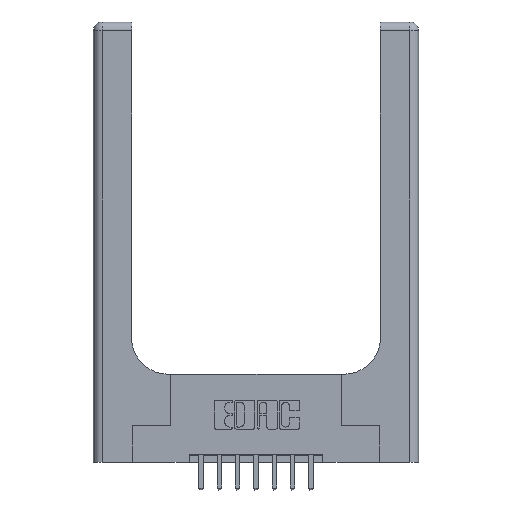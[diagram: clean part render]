
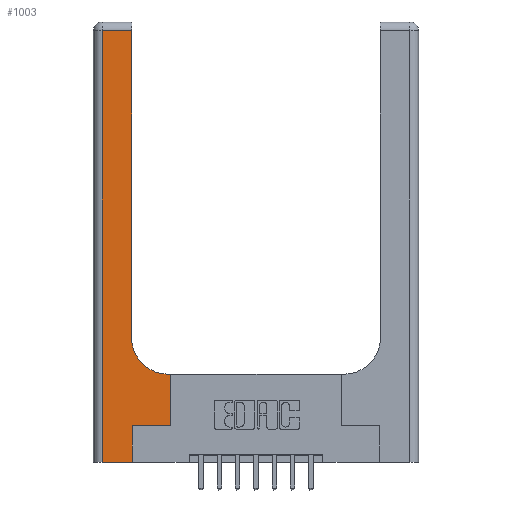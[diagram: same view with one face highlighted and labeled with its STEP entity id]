
A CAD part, top view. The second image highlights one B-rep face of the part: STEP entity #1003.
In plain terms, the highlighted planar face has unit normal (0, 0, 1).
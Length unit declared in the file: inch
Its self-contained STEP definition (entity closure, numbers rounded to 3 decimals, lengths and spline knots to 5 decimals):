
#156 = CARTESIAN_POINT ( 'NONE',  ( 0.51, 0.85, 0.37 ) ) ;
#157 = LINE ( 'NONE', #9259, #11962 ) ;
#174 = VECTOR ( 'NONE', #3947, 39.37008 ) ;
#185 = DIRECTION ( 'NONE',  ( 0., 1., 0. ) ) ;
#489 = VERTEX_POINT ( 'NONE', #7079 ) ;
#1003 = ADVANCED_FACE ( 'NONE', ( #2369 ), #7775, .F. ) ;
#1210 = CARTESIAN_POINT ( 'NONE',  ( 0.265, 0.25, 0.37 ) ) ;
#1618 = LINE ( 'NONE', #1210, #6389 ) ;
#1628 = EDGE_CURVE ( 'NONE', #11171, #5845, #3055, .T. ) ;
#1662 = VERTEX_POINT ( 'NONE', #12021 ) ;
#1709 = DIRECTION ( 'NONE',  ( 0., -1., 0. ) ) ;
#1974 = DIRECTION ( 'NONE',  ( 1., 0., 0. ) ) ;
#2057 = CARTESIAN_POINT ( 'NONE',  ( 0.51, 0.6, 0.37 ) ) ;
#2179 = VECTOR ( 'NONE', #1974, 39.37008 ) ;
#2369 = FACE_OUTER_BOUND ( 'NONE', #11499, .T. ) ;
#2443 = DIRECTION ( 'NONE',  ( 1., 0., 0. ) ) ;
#2657 = LINE ( 'NONE', #5059, #6920 ) ;
#2875 = LINE ( 'NONE', #8528, #2179 ) ;
#2930 = LINE ( 'NONE', #10883, #8245 ) ;
#3055 = LINE ( 'NONE', #8002, #6440 ) ;
#3266 = VERTEX_POINT ( 'NONE', #8598 ) ;
#3276 = CARTESIAN_POINT ( 'NONE',  ( 0., 3., 0.37 ) ) ;
#3330 = ORIENTED_EDGE ( 'NONE', *, *, #7799, .T. ) ;
#3516 = EDGE_CURVE ( 'NONE', #12905, #3266, #2657, .T. ) ;
#3571 = ORIENTED_EDGE ( 'NONE', *, *, #1628, .T. ) ;
#3836 = ORIENTED_EDGE ( 'NONE', *, *, #6866, .T. ) ;
#3947 = DIRECTION ( 'NONE',  ( -1., 0., 0. ) ) ;
#4151 = CARTESIAN_POINT ( 'NONE',  ( 0., 2.94, 0.37 ) ) ;
#4368 = DIRECTION ( 'NONE',  ( 0., 1., 0. ) ) ;
#4957 = LINE ( 'NONE', #4151, #174 ) ;
#5059 = CARTESIAN_POINT ( 'NONE',  ( 0.06, 3., 0.37 ) ) ;
#5617 = VERTEX_POINT ( 'NONE', #11482 ) ;
#5618 = DIRECTION ( 'NONE',  ( 1., 0., 0. ) ) ;
#5726 = VERTEX_POINT ( 'NONE', #13419 ) ;
#5845 = VERTEX_POINT ( 'NONE', #13540 ) ;
#6379 = EDGE_CURVE ( 'NONE', #3266, #5617, #2875, .T. ) ;
#6389 = VECTOR ( 'NONE', #5618, 39.37008 ) ;
#6440 = VECTOR ( 'NONE', #185, 39.37008 ) ;
#6866 = EDGE_CURVE ( 'NONE', #489, #9296, #9216, .T. ) ;
#6920 = VECTOR ( 'NONE', #1709, 39.37008 ) ;
#7079 = CARTESIAN_POINT ( 'NONE',  ( 0.528, 0.6, 0.37 ) ) ;
#7583 = EDGE_CURVE ( 'NONE', #5726, #1662, #1618, .T. ) ;
#7775 = PLANE ( 'NONE',  #13805 ) ;
#7799 = EDGE_CURVE ( 'NONE', #5845, #12905, #4957, .T. ) ;
#7831 = VECTOR ( 'NONE', #9234, 39.37008 ) ;
#8002 = CARTESIAN_POINT ( 'NONE',  ( 0.26, 3., 0.37 ) ) ;
#8194 = EDGE_CURVE ( 'NONE', #5617, #5726, #157, .T. ) ;
#8245 = VECTOR ( 'NONE', #4368, 39.37008 ) ;
#8502 = CARTESIAN_POINT ( 'NONE',  ( 0.26, 0.85, 0.37 ) ) ;
#8528 = CARTESIAN_POINT ( 'NONE',  ( 0., 0., 0.37 ) ) ;
#8598 = CARTESIAN_POINT ( 'NONE',  ( 0.06, 0., 0.37 ) ) ;
#9134 = CIRCLE ( 'NONE', #13673, 0.25 ) ;
#9216 = LINE ( 'NONE', #11328, #7831 ) ;
#9234 = DIRECTION ( 'NONE',  ( -1., 0., 0. ) ) ;
#9259 = CARTESIAN_POINT ( 'NONE',  ( 0.265, 0., 0.37 ) ) ;
#9296 = VERTEX_POINT ( 'NONE', #2057 ) ;
#9601 = CARTESIAN_POINT ( 'NONE',  ( 0.06, 2.94, 0.37 ) ) ;
#10428 = DIRECTION ( 'NONE',  ( 0., 1., 0. ) ) ;
#10652 = EDGE_CURVE ( 'NONE', #9296, #11171, #9134, .T. ) ;
#10883 = CARTESIAN_POINT ( 'NONE',  ( 0.528, 0.25, 0.37 ) ) ;
#10963 = ORIENTED_EDGE ( 'NONE', *, *, #7583, .T. ) ;
#11143 = DIRECTION ( 'NONE',  ( 0., 0., -1. ) ) ;
#11171 = VERTEX_POINT ( 'NONE', #8502 ) ;
#11328 = CARTESIAN_POINT ( 'NONE',  ( 0.26, 0.6, 0.37 ) ) ;
#11482 = CARTESIAN_POINT ( 'NONE',  ( 0.265, 0., 0.37 ) ) ;
#11499 = EDGE_LOOP ( 'NONE', ( #3571, #3330, #11743, #14583, #13889, #10963, #14199, #3836, #12046 ) ) ;
#11743 = ORIENTED_EDGE ( 'NONE', *, *, #3516, .T. ) ;
#11962 = VECTOR ( 'NONE', #10428, 39.37008 ) ;
#12021 = CARTESIAN_POINT ( 'NONE',  ( 0.528, 0.25, 0.37 ) ) ;
#12046 = ORIENTED_EDGE ( 'NONE', *, *, #10652, .T. ) ;
#12263 = DIRECTION ( 'NONE',  ( -1., 0., 0. ) ) ;
#12905 = VERTEX_POINT ( 'NONE', #9601 ) ;
#13233 = EDGE_CURVE ( 'NONE', #1662, #489, #2930, .T. ) ;
#13419 = CARTESIAN_POINT ( 'NONE',  ( 0.265, 0.25, 0.37 ) ) ;
#13540 = CARTESIAN_POINT ( 'NONE',  ( 0.26, 2.94, 0.37 ) ) ;
#13672 = DIRECTION ( 'NONE',  ( 0., 0., -1. ) ) ;
#13673 = AXIS2_PLACEMENT_3D ( 'NONE', #156, #13672, #2443 ) ;
#13805 = AXIS2_PLACEMENT_3D ( 'NONE', #3276, #11143, #12263 ) ;
#13889 = ORIENTED_EDGE ( 'NONE', *, *, #8194, .T. ) ;
#14199 = ORIENTED_EDGE ( 'NONE', *, *, #13233, .T. ) ;
#14583 = ORIENTED_EDGE ( 'NONE', *, *, #6379, .T. ) ;
